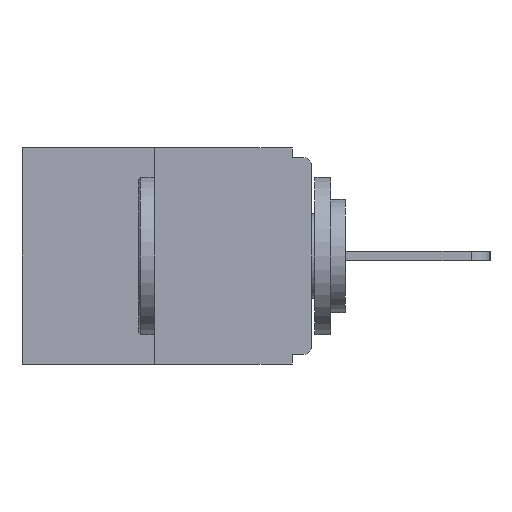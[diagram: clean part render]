
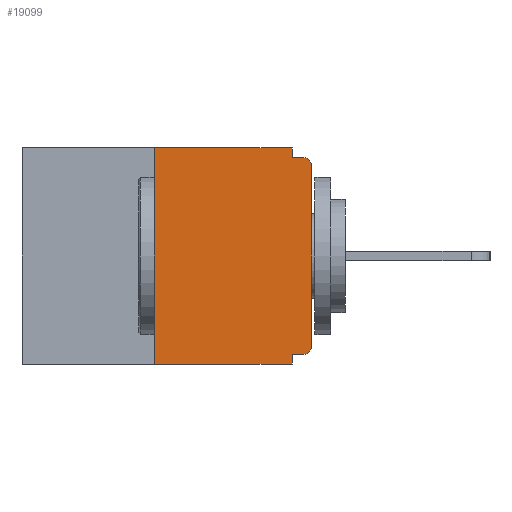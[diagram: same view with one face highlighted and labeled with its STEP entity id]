
A CAD part, left-side view. The second image highlights one B-rep face of the part: STEP entity #19099.
In plain terms, the highlighted planar face has unit normal (-1, 0, 0).
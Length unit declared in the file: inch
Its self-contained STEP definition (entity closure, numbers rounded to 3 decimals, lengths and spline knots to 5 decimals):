
#129 = CARTESIAN_POINT ( 'NONE',  ( 0., 0., -0.015 ) ) ;
#375 = VECTOR ( 'NONE', #14951, 39.37008 ) ;
#461 = ORIENTED_EDGE ( 'NONE', *, *, #18970, .F. ) ;
#757 = VERTEX_POINT ( 'NONE', #9819 ) ;
#825 = CARTESIAN_POINT ( 'NONE',  ( 0., 0.015, -0.03 ) ) ;
#1028 = VECTOR ( 'NONE', #18979, 39.37008 ) ;
#1235 = CARTESIAN_POINT ( 'NONE',  ( 0., 0.015, -0.015 ) ) ;
#1516 = ORIENTED_EDGE ( 'NONE', *, *, #5751, .F. ) ;
#1557 = CARTESIAN_POINT ( 'NONE',  ( 0., 0.46, -0.343 ) ) ;
#1601 = DIRECTION ( 'NONE',  ( 0., 0., -1. ) ) ;
#1680 = CARTESIAN_POINT ( 'NONE',  ( 0., 0., -0.328 ) ) ;
#2044 = CARTESIAN_POINT ( 'NONE',  ( 0., 0.031, -0.343 ) ) ;
#2553 = VECTOR ( 'NONE', #16289, 39.37008 ) ;
#2889 = CARTESIAN_POINT ( 'NONE',  ( 0., 0.46, 0. ) ) ;
#3228 = CARTESIAN_POINT ( 'NONE',  ( 0., 0.031, -0.015 ) ) ;
#3335 = ORIENTED_EDGE ( 'NONE', *, *, #22022, .T. ) ;
#3458 = DIRECTION ( 'NONE',  ( -1., 0., 0. ) ) ;
#3510 = CARTESIAN_POINT ( 'NONE',  ( 0., 0.031, -0.328 ) ) ;
#3838 = CARTESIAN_POINT ( 'NONE',  ( 0., 0.031, -0.343 ) ) ;
#3982 = DIRECTION ( 'NONE',  ( 0., -1., 0. ) ) ;
#4195 = AXIS2_PLACEMENT_3D ( 'NONE', #2889, #19598, #15764 ) ;
#5564 = DIRECTION ( 'NONE',  ( 0., 0., -1. ) ) ;
#5751 = EDGE_CURVE ( 'NONE', #8038, #20318, #7397, .T. ) ;
#6859 = DIRECTION ( 'NONE',  ( 0., 0., -1. ) ) ;
#6958 = VECTOR ( 'NONE', #3982, 39.37008 ) ;
#6983 = EDGE_LOOP ( 'NONE', ( #461, #23455, #3335, #1516, #22411, #16066, #22956, #20066, #22189, #8412 ) ) ;
#7083 = VERTEX_POINT ( 'NONE', #1235 ) ;
#7175 = VERTEX_POINT ( 'NONE', #7502 ) ;
#7397 = LINE ( 'NONE', #3838, #17319 ) ;
#7502 = CARTESIAN_POINT ( 'NONE',  ( 0., 0., -0.313 ) ) ;
#8002 = EDGE_CURVE ( 'NONE', #21679, #7083, #24153, .T. ) ;
#8038 = VERTEX_POINT ( 'NONE', #3510 ) ;
#8412 = ORIENTED_EDGE ( 'NONE', *, *, #20288, .F. ) ;
#8556 = LINE ( 'NONE', #1557, #21605 ) ;
#8916 = DIRECTION ( 'NONE',  ( 0., -1., 0. ) ) ;
#9284 = CARTESIAN_POINT ( 'NONE',  ( 0., 0.25, 0. ) ) ;
#9368 = CARTESIAN_POINT ( 'NONE',  ( 0., 0.015, -0.328 ) ) ;
#9419 = DIRECTION ( 'NONE',  ( 0., 0., -1. ) ) ;
#9819 = CARTESIAN_POINT ( 'NONE',  ( 0., 0.25, -0.343 ) ) ;
#10946 = CARTESIAN_POINT ( 'NONE',  ( 0., 0.031, 0. ) ) ;
#11395 = CARTESIAN_POINT ( 'NONE',  ( 0., 0.031, 0. ) ) ;
#11452 = VERTEX_POINT ( 'NONE', #10946 ) ;
#12037 = EDGE_CURVE ( 'NONE', #7175, #16723, #24323, .T. ) ;
#12047 = AXIS2_PLACEMENT_3D ( 'NONE', #22722, #3458, #1601 ) ;
#12115 = FACE_OUTER_BOUND ( 'NONE', #6983, .T. ) ;
#13963 = DIRECTION ( 'NONE',  ( -1., 0., 0. ) ) ;
#14174 = PLANE ( 'NONE',  #4195 ) ;
#14398 = EDGE_CURVE ( 'NONE', #23240, #8038, #20243, .T. ) ;
#14423 = CIRCLE ( 'NONE', #17551, 0.015 ) ;
#14698 = LINE ( 'NONE', #9284, #2553 ) ;
#14948 = EDGE_CURVE ( 'NONE', #23240, #7175, #23847, .T. ) ;
#14951 = DIRECTION ( 'NONE',  ( 0., 0., 1. ) ) ;
#15764 = DIRECTION ( 'NONE',  ( 0., 0., -1. ) ) ;
#16066 = ORIENTED_EDGE ( 'NONE', *, *, #14948, .T. ) ;
#16289 = DIRECTION ( 'NONE',  ( 0., 0., 1. ) ) ;
#16723 = VERTEX_POINT ( 'NONE', #21539 ) ;
#17319 = VECTOR ( 'NONE', #5564, 39.37008 ) ;
#17551 = AXIS2_PLACEMENT_3D ( 'NONE', #825, #13963, #6859 ) ;
#18758 = VECTOR ( 'NONE', #9419, 39.37008 ) ;
#18827 = CARTESIAN_POINT ( 'NONE',  ( 0., 0.25, 0. ) ) ;
#18832 = EDGE_CURVE ( 'NONE', #757, #21361, #14698, .T. ) ;
#18970 = EDGE_CURVE ( 'NONE', #21361, #11452, #22715, .T. ) ;
#18979 = DIRECTION ( 'NONE',  ( 0., -1., 0. ) ) ;
#19098 = LINE ( 'NONE', #11395, #18758 ) ;
#19099 = ADVANCED_FACE ( 'NONE', ( #12115 ), #14174, .F. ) ;
#19598 = DIRECTION ( 'NONE',  ( 1., 0., 0. ) ) ;
#19878 = EDGE_CURVE ( 'NONE', #16723, #7083, #14423, .T. ) ;
#20066 = ORIENTED_EDGE ( 'NONE', *, *, #19878, .T. ) ;
#20243 = LINE ( 'NONE', #1680, #23435 ) ;
#20288 = EDGE_CURVE ( 'NONE', #11452, #21679, #19098, .T. ) ;
#20318 = VERTEX_POINT ( 'NONE', #2044 ) ;
#21361 = VERTEX_POINT ( 'NONE', #18827 ) ;
#21539 = CARTESIAN_POINT ( 'NONE',  ( 0., 0., -0.03 ) ) ;
#21605 = VECTOR ( 'NONE', #8916, 39.37008 ) ;
#21679 = VERTEX_POINT ( 'NONE', #3228 ) ;
#22022 = EDGE_CURVE ( 'NONE', #757, #20318, #8556, .T. ) ;
#22122 = DIRECTION ( 'NONE',  ( 0., 1., 0. ) ) ;
#22189 = ORIENTED_EDGE ( 'NONE', *, *, #8002, .F. ) ;
#22371 = CARTESIAN_POINT ( 'NONE',  ( 0., 0., 0. ) ) ;
#22411 = ORIENTED_EDGE ( 'NONE', *, *, #14398, .F. ) ;
#22479 = CARTESIAN_POINT ( 'NONE',  ( 0., 0.46, 0. ) ) ;
#22715 = LINE ( 'NONE', #22479, #1028 ) ;
#22722 = CARTESIAN_POINT ( 'NONE',  ( 0., 0.015, -0.313 ) ) ;
#22956 = ORIENTED_EDGE ( 'NONE', *, *, #12037, .T. ) ;
#23240 = VERTEX_POINT ( 'NONE', #9368 ) ;
#23435 = VECTOR ( 'NONE', #22122, 39.37008 ) ;
#23455 = ORIENTED_EDGE ( 'NONE', *, *, #18832, .F. ) ;
#23847 = CIRCLE ( 'NONE', #12047, 0.015 ) ;
#24153 = LINE ( 'NONE', #129, #6958 ) ;
#24323 = LINE ( 'NONE', #22371, #375 ) ;
